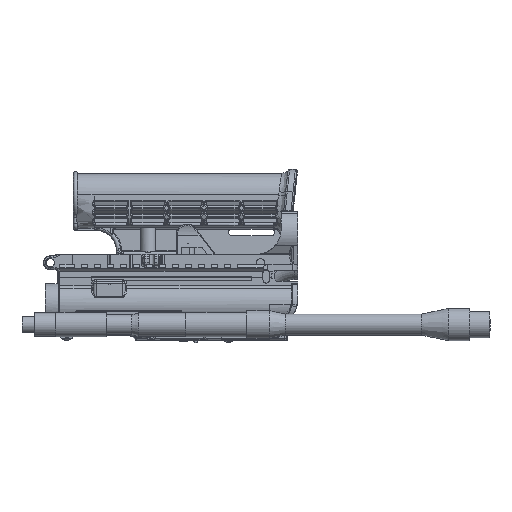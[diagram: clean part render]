
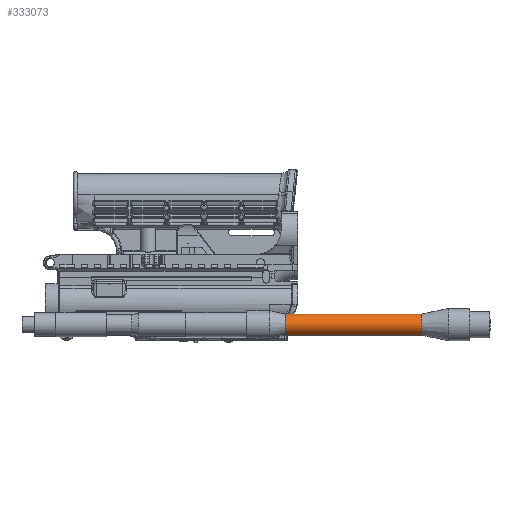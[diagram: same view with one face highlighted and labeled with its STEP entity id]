
A CAD part, top view. The second image highlights one B-rep face of the part: STEP entity #333073.
In plain terms, the highlighted cylindrical face has radius 8.128 mm (diameter 16.256 mm), a full revolution.
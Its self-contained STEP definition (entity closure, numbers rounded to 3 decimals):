
#28449 = CARTESIAN_POINT ( 'NONE',  ( 37.084, 0., 0. ) ) ;
#37600 = DIRECTION ( 'NONE',  ( -1., 0., 0. ) ) ;
#72232 = CIRCLE ( 'NONE', #247367, 8.128 ) ;
#76823 = CYLINDRICAL_SURFACE ( 'NONE', #246789, 8.128 ) ;
#79674 = DIRECTION ( 'NONE',  ( -1., 0., 0. ) ) ;
#100106 = EDGE_LOOP ( 'NONE', ( #257425 ) ) ;
#118226 = FACE_OUTER_BOUND ( 'NONE', #100106, .T. ) ;
#130950 = FACE_OUTER_BOUND ( 'NONE', #252440, .T. ) ;
#133224 = DIRECTION ( 'NONE',  ( 0., -1., 0. ) ) ;
#139565 = CIRCLE ( 'NONE', #243369, 8.128 ) ;
#156617 = VERTEX_POINT ( 'NONE', #212486 ) ;
#196893 = CARTESIAN_POINT ( 'NONE',  ( 141.986, 0., 0. ) ) ;
#207068 = EDGE_CURVE ( 'NONE', #248248, #248248, #139565, .T. ) ;
#212486 = CARTESIAN_POINT ( 'NONE',  ( 141.986, 8.128, 0. ) ) ;
#237162 = ORIENTED_EDGE ( 'NONE', *, *, #306668, .T. ) ;
#240613 = DIRECTION ( 'NONE',  ( 0., 1., 0. ) ) ;
#243369 = AXIS2_PLACEMENT_3D ( 'NONE', #28449, #79674, #133224 ) ;
#246789 = AXIS2_PLACEMENT_3D ( 'NONE', #196893, #37600, #278206 ) ;
#247367 = AXIS2_PLACEMENT_3D ( 'NONE', #320808, #319650, #240613 ) ;
#248248 = VERTEX_POINT ( 'NONE', #313710 ) ;
#252440 = EDGE_LOOP ( 'NONE', ( #237162 ) ) ;
#257425 = ORIENTED_EDGE ( 'NONE', *, *, #207068, .F. ) ;
#278206 = DIRECTION ( 'NONE',  ( 0., 0., 1. ) ) ;
#306668 = EDGE_CURVE ( 'NONE', #156617, #156617, #72232, .T. ) ;
#313710 = CARTESIAN_POINT ( 'NONE',  ( 37.084, -8.128, 0. ) ) ;
#319650 = DIRECTION ( 'NONE',  ( -1., 0., 0. ) ) ;
#320808 = CARTESIAN_POINT ( 'NONE',  ( 141.986, 0., 0. ) ) ;
#333073 = ADVANCED_FACE ( 'NONE', ( #130950, #118226 ), #76823, .T. ) ;
